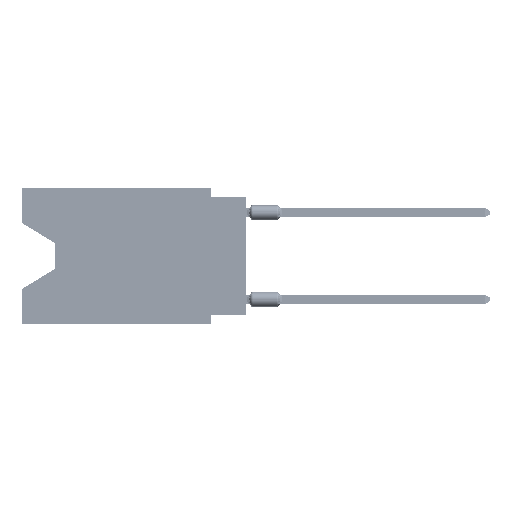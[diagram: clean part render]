
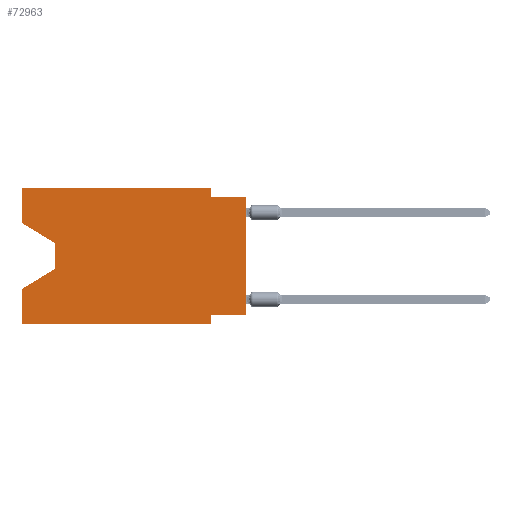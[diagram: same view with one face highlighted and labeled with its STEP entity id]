
A CAD part, left-side view. The second image highlights one B-rep face of the part: STEP entity #72963.
In plain terms, the highlighted planar face has unit normal (-1, 0, 0).
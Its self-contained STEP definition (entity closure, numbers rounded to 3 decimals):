
#598 = LINE ( 'NONE', #26274, #36381 ) ;
#676 = CARTESIAN_POINT ( 'NONE',  ( 0., 16.383, 0. ) ) ;
#1312 = LINE ( 'NONE', #64794, #13771 ) ;
#1587 = EDGE_CURVE ( 'NONE', #43508, #4457, #61710, .T. ) ;
#3445 = EDGE_CURVE ( 'NONE', #38875, #19036, #69617, .T. ) ;
#4097 = EDGE_CURVE ( 'NONE', #38825, #40167, #42950, .T. ) ;
#4457 = VERTEX_POINT ( 'NONE', #64788 ) ;
#4467 = LINE ( 'NONE', #81785, #73769 ) ;
#5466 = VECTOR ( 'NONE', #57371, 1000. ) ;
#7596 = EDGE_CURVE ( 'NONE', #34942, #38663, #7811, .T. ) ;
#7811 = LINE ( 'NONE', #676, #75945 ) ;
#8374 = DIRECTION ( 'NONE',  ( 0., -1., 0. ) ) ;
#8823 = VERTEX_POINT ( 'NONE', #53603 ) ;
#10852 = DIRECTION ( 'NONE',  ( 0., 0.855, -0.519 ) ) ;
#12835 = CARTESIAN_POINT ( 'NONE',  ( 0., 0., -0.635 ) ) ;
#12923 = CARTESIAN_POINT ( 'NONE',  ( 0., 16.383, 0. ) ) ;
#13445 = LINE ( 'NONE', #52496, #31515 ) ;
#13482 = VECTOR ( 'NONE', #66685, 1000. ) ;
#13771 = VECTOR ( 'NONE', #40387, 1000. ) ;
#15099 = ORIENTED_EDGE ( 'NONE', *, *, #4097, .T. ) ;
#15699 = CARTESIAN_POINT ( 'NONE',  ( 0., 16.383, -2.546 ) ) ;
#16875 = ORIENTED_EDGE ( 'NONE', *, *, #3445, .F. ) ;
#17513 = EDGE_CURVE ( 'NONE', #45130, #38875, #598, .T. ) ;
#18698 = CARTESIAN_POINT ( 'NONE',  ( 0., 16.383, 0. ) ) ;
#19036 = VERTEX_POINT ( 'NONE', #59494 ) ;
#19621 = CARTESIAN_POINT ( 'NONE',  ( 0., 0., 0. ) ) ;
#20714 = CARTESIAN_POINT ( 'NONE',  ( 0., 2.54, -0.635 ) ) ;
#22544 = CARTESIAN_POINT ( 'NONE',  ( 0., 2.54, 0. ) ) ;
#23686 = EDGE_CURVE ( 'NONE', #8823, #4457, #46865, .T. ) ;
#24751 = CARTESIAN_POINT ( 'NONE',  ( 0., 0., -0.635 ) ) ;
#26274 = CARTESIAN_POINT ( 'NONE',  ( 0., 0., -9.271 ) ) ;
#29154 = DIRECTION ( 'NONE',  ( 0., -0.855, -0.519 ) ) ;
#29252 = ORIENTED_EDGE ( 'NONE', *, *, #71741, .T. ) ;
#30436 = ORIENTED_EDGE ( 'NONE', *, *, #1587, .T. ) ;
#30720 = EDGE_CURVE ( 'NONE', #8823, #19036, #13445, .T. ) ;
#30745 = ORIENTED_EDGE ( 'NONE', *, *, #36192, .F. ) ;
#31515 = VECTOR ( 'NONE', #8374, 1000. ) ;
#32687 = DIRECTION ( 'NONE',  ( 1., 0., 0. ) ) ;
#33002 = VECTOR ( 'NONE', #46056, 1000. ) ;
#34111 = VECTOR ( 'NONE', #38107, 1000. ) ;
#34942 = VERTEX_POINT ( 'NONE', #18698 ) ;
#36192 = EDGE_CURVE ( 'NONE', #37917, #58230, #57778, .T. ) ;
#36381 = VECTOR ( 'NONE', #51871, 1000. ) ;
#36562 = CARTESIAN_POINT ( 'NONE',  ( 0., 0., -9.271 ) ) ;
#37688 = CARTESIAN_POINT ( 'NONE',  ( 0., 2.54, -9.906 ) ) ;
#37917 = VERTEX_POINT ( 'NONE', #20714 ) ;
#38107 = DIRECTION ( 'NONE',  ( 0., 0., -1. ) ) ;
#38663 = VERTEX_POINT ( 'NONE', #73150 ) ;
#38825 = VERTEX_POINT ( 'NONE', #81500 ) ;
#38875 = VERTEX_POINT ( 'NONE', #78537 ) ;
#39190 = VECTOR ( 'NONE', #10852, 1000. ) ;
#39853 = EDGE_CURVE ( 'NONE', #38825, #34942, #1312, .T. ) ;
#40167 = VERTEX_POINT ( 'NONE', #72658 ) ;
#40387 = DIRECTION ( 'NONE',  ( 0., 0., 1. ) ) ;
#40592 = DIRECTION ( 'NONE',  ( 0., -1., 0. ) ) ;
#42950 = LINE ( 'NONE', #15699, #58318 ) ;
#43508 = VERTEX_POINT ( 'NONE', #69496 ) ;
#45130 = VERTEX_POINT ( 'NONE', #36562 ) ;
#45254 = DIRECTION ( 'NONE',  ( 0., 0., 1. ) ) ;
#45272 = PLANE ( 'NONE',  #77797 ) ;
#45529 = EDGE_CURVE ( 'NONE', #40167, #43508, #4467, .T. ) ;
#46056 = DIRECTION ( 'NONE',  ( 0., 0., 1. ) ) ;
#46865 = LINE ( 'NONE', #78001, #33002 ) ;
#49437 = DIRECTION ( 'NONE',  ( 0., 0., -1. ) ) ;
#51871 = DIRECTION ( 'NONE',  ( 0., 1., 0. ) ) ;
#52496 = CARTESIAN_POINT ( 'NONE',  ( 0., 16.383, -9.906 ) ) ;
#53603 = CARTESIAN_POINT ( 'NONE',  ( 0., 16.383, -9.906 ) ) ;
#54969 = CARTESIAN_POINT ( 'NONE',  ( 0., 13.97, -5.893 ) ) ;
#55619 = EDGE_LOOP ( 'NONE', ( #15099, #57682, #30436, #56198, #70274, #16875, #70697, #29252, #30745, #74232, #73278, #73091 ) ) ;
#56198 = ORIENTED_EDGE ( 'NONE', *, *, #23686, .F. ) ;
#57371 = DIRECTION ( 'NONE',  ( 0., -1., 0. ) ) ;
#57453 = DIRECTION ( 'NONE',  ( 0., 0., -1. ) ) ;
#57682 = ORIENTED_EDGE ( 'NONE', *, *, #45529, .T. ) ;
#57778 = LINE ( 'NONE', #12835, #5466 ) ;
#58230 = VERTEX_POINT ( 'NONE', #24751 ) ;
#58318 = VECTOR ( 'NONE', #29154, 1000. ) ;
#59494 = CARTESIAN_POINT ( 'NONE',  ( 0., 2.54, -9.906 ) ) ;
#61607 = LINE ( 'NONE', #22544, #13482 ) ;
#61710 = LINE ( 'NONE', #54969, #39190 ) ;
#64788 = CARTESIAN_POINT ( 'NONE',  ( 0., 16.383, -7.36 ) ) ;
#64794 = CARTESIAN_POINT ( 'NONE',  ( 0., 16.383, 0. ) ) ;
#66685 = DIRECTION ( 'NONE',  ( 0., 0., -1. ) ) ;
#69496 = CARTESIAN_POINT ( 'NONE',  ( 0., 13.97, -5.893 ) ) ;
#69617 = LINE ( 'NONE', #37688, #34111 ) ;
#70274 = ORIENTED_EDGE ( 'NONE', *, *, #30720, .T. ) ;
#70490 = FACE_OUTER_BOUND ( 'NONE', #55619, .T. ) ;
#70697 = ORIENTED_EDGE ( 'NONE', *, *, #17513, .F. ) ;
#71741 = EDGE_CURVE ( 'NONE', #45130, #58230, #77196, .T. ) ;
#72658 = CARTESIAN_POINT ( 'NONE',  ( 0., 13.97, -4.013 ) ) ;
#72963 = ADVANCED_FACE ( 'NONE', ( #70490 ), #45272, .F. ) ;
#73091 = ORIENTED_EDGE ( 'NONE', *, *, #39853, .F. ) ;
#73150 = CARTESIAN_POINT ( 'NONE',  ( 0., 2.54, 0. ) ) ;
#73278 = ORIENTED_EDGE ( 'NONE', *, *, #7596, .F. ) ;
#73769 = VECTOR ( 'NONE', #49437, 1000. ) ;
#74232 = ORIENTED_EDGE ( 'NONE', *, *, #75255, .F. ) ;
#75255 = EDGE_CURVE ( 'NONE', #38663, #37917, #61607, .T. ) ;
#75945 = VECTOR ( 'NONE', #40592, 1000. ) ;
#77196 = LINE ( 'NONE', #19621, #80297 ) ;
#77797 = AXIS2_PLACEMENT_3D ( 'NONE', #12923, #32687, #57453 ) ;
#78001 = CARTESIAN_POINT ( 'NONE',  ( 0., 16.383, 0. ) ) ;
#78537 = CARTESIAN_POINT ( 'NONE',  ( 0., 2.54, -9.271 ) ) ;
#80297 = VECTOR ( 'NONE', #45254, 1000. ) ;
#81500 = CARTESIAN_POINT ( 'NONE',  ( 0., 16.383, -2.546 ) ) ;
#81785 = CARTESIAN_POINT ( 'NONE',  ( 0., 13.97, -4.013 ) ) ;
